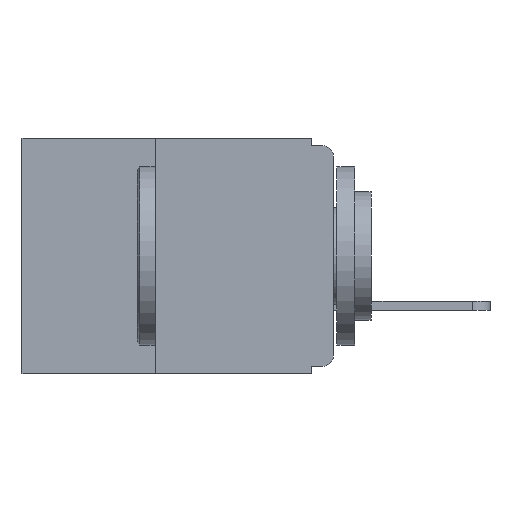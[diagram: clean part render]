
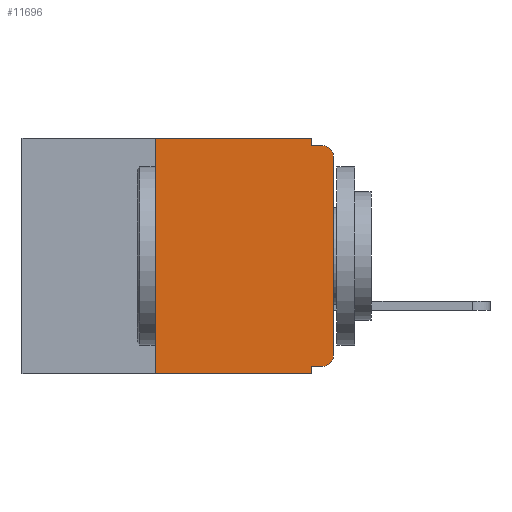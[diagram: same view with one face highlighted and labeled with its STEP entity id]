
A CAD part, left-side view. The second image highlights one B-rep face of the part: STEP entity #11696.
In plain terms, the highlighted planar face has unit normal (-1, 0, 0).
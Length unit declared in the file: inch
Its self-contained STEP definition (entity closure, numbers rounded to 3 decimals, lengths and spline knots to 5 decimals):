
#84 = EDGE_CURVE ( 'NONE', #11454, #4569, #12786, .T. ) ;
#391 = CARTESIAN_POINT ( 'NONE',  ( 0., 0., 0. ) ) ;
#518 = VECTOR ( 'NONE', #15742, 39.37008 ) ;
#551 = VERTEX_POINT ( 'NONE', #2414 ) ;
#1000 = LINE ( 'NONE', #11585, #13023 ) ;
#1158 = EDGE_CURVE ( 'NONE', #9826, #9682, #7906, .T. ) ;
#1329 = CARTESIAN_POINT ( 'NONE',  ( 0., 0.031, -0.33 ) ) ;
#1333 = VECTOR ( 'NONE', #4972, 39.37008 ) ;
#1735 = AXIS2_PLACEMENT_3D ( 'NONE', #10075, #7934, #3532 ) ;
#1920 = EDGE_CURVE ( 'NONE', #6484, #8667, #3217, .T. ) ;
#2244 = CARTESIAN_POINT ( 'NONE',  ( 0., 0., -0.32 ) ) ;
#2414 = CARTESIAN_POINT ( 'NONE',  ( 0., 0.25, -0.33 ) ) ;
#2590 = VECTOR ( 'NONE', #13302, 39.37008 ) ;
#3217 = CIRCLE ( 'NONE', #10642, 0.015 ) ;
#3390 = CARTESIAN_POINT ( 'NONE',  ( 0., 0.015, -0.32 ) ) ;
#3454 = EDGE_CURVE ( 'NONE', #6484, #11454, #14997, .T. ) ;
#3532 = DIRECTION ( 'NONE',  ( 0., 0., -1. ) ) ;
#4244 = DIRECTION ( 'NONE',  ( 0., 0., -1. ) ) ;
#4375 = ORIENTED_EDGE ( 'NONE', *, *, #4645, .F. ) ;
#4415 = CARTESIAN_POINT ( 'NONE',  ( 0., 0.015, -0.305 ) ) ;
#4519 = CARTESIAN_POINT ( 'NONE',  ( 0., 0.25, 0. ) ) ;
#4569 = VERTEX_POINT ( 'NONE', #1329 ) ;
#4645 = EDGE_CURVE ( 'NONE', #9682, #10896, #1000, .T. ) ;
#4791 = ORIENTED_EDGE ( 'NONE', *, *, #10527, .T. ) ;
#4972 = DIRECTION ( 'NONE',  ( 0., -1., 0. ) ) ;
#5139 = ORIENTED_EDGE ( 'NONE', *, *, #84, .F. ) ;
#6115 = LINE ( 'NONE', #10929, #11554 ) ;
#6153 = FACE_OUTER_BOUND ( 'NONE', #7063, .T. ) ;
#6484 = VERTEX_POINT ( 'NONE', #3390 ) ;
#6766 = CARTESIAN_POINT ( 'NONE',  ( 0., 0.437, -0.33 ) ) ;
#7063 = EDGE_LOOP ( 'NONE', ( #11499, #4791, #9771, #4375, #14673, #13803, #12579, #5139, #9735, #7335 ) ) ;
#7159 = DIRECTION ( 'NONE',  ( 0., 0., -1. ) ) ;
#7201 = PLANE ( 'NONE',  #1735 ) ;
#7335 = ORIENTED_EDGE ( 'NONE', *, *, #1920, .T. ) ;
#7432 = CARTESIAN_POINT ( 'NONE',  ( 0., 0.031, -0.33 ) ) ;
#7902 = DIRECTION ( 'NONE',  ( 0., -1., 0. ) ) ;
#7906 = LINE ( 'NONE', #10744, #518 ) ;
#7934 = DIRECTION ( 'NONE',  ( 1., 0., 0. ) ) ;
#7978 = VECTOR ( 'NONE', #13998, 39.37008 ) ;
#8246 = CARTESIAN_POINT ( 'NONE',  ( 0., 0.031, -0.01 ) ) ;
#8367 = DIRECTION ( 'NONE',  ( -1., 0., 0. ) ) ;
#8544 = CIRCLE ( 'NONE', #11048, 0.015 ) ;
#8584 = DIRECTION ( 'NONE',  ( 0., 0., 1. ) ) ;
#8633 = DIRECTION ( 'NONE',  ( 0., 0., -1. ) ) ;
#8667 = VERTEX_POINT ( 'NONE', #10790 ) ;
#8693 = CARTESIAN_POINT ( 'NONE',  ( 0., 0.015, -0.025 ) ) ;
#8848 = CARTESIAN_POINT ( 'NONE',  ( 0., 0., -0.01 ) ) ;
#9064 = CARTESIAN_POINT ( 'NONE',  ( 0., 0., -0.025 ) ) ;
#9523 = VECTOR ( 'NONE', #8633, 39.37008 ) ;
#9682 = VERTEX_POINT ( 'NONE', #15117 ) ;
#9735 = ORIENTED_EDGE ( 'NONE', *, *, #3454, .F. ) ;
#9771 = ORIENTED_EDGE ( 'NONE', *, *, #10522, .F. ) ;
#9826 = VERTEX_POINT ( 'NONE', #4519 ) ;
#9944 = DIRECTION ( 'NONE',  ( -1., 0., 0. ) ) ;
#10005 = EDGE_CURVE ( 'NONE', #8667, #11952, #14163, .T. ) ;
#10075 = CARTESIAN_POINT ( 'NONE',  ( 0., 0.437, 0. ) ) ;
#10522 = EDGE_CURVE ( 'NONE', #10896, #11429, #14916, .T. ) ;
#10527 = EDGE_CURVE ( 'NONE', #11952, #11429, #8544, .T. ) ;
#10573 = LINE ( 'NONE', #6766, #13062 ) ;
#10642 = AXIS2_PLACEMENT_3D ( 'NONE', #4415, #8367, #7159 ) ;
#10744 = CARTESIAN_POINT ( 'NONE',  ( 0., 0.437, 0. ) ) ;
#10790 = CARTESIAN_POINT ( 'NONE',  ( 0., 0., -0.305 ) ) ;
#10896 = VERTEX_POINT ( 'NONE', #8246 ) ;
#10929 = CARTESIAN_POINT ( 'NONE',  ( 0., 0.25, -0.33 ) ) ;
#11048 = AXIS2_PLACEMENT_3D ( 'NONE', #8693, #9944, #11182 ) ;
#11182 = DIRECTION ( 'NONE',  ( 0., 0., -1. ) ) ;
#11429 = VERTEX_POINT ( 'NONE', #12475 ) ;
#11454 = VERTEX_POINT ( 'NONE', #12737 ) ;
#11499 = ORIENTED_EDGE ( 'NONE', *, *, #10005, .T. ) ;
#11554 = VECTOR ( 'NONE', #8584, 39.37008 ) ;
#11585 = CARTESIAN_POINT ( 'NONE',  ( 0., 0.031, 0. ) ) ;
#11696 = ADVANCED_FACE ( 'NONE', ( #6153 ), #7201, .F. ) ;
#11952 = VERTEX_POINT ( 'NONE', #9064 ) ;
#12475 = CARTESIAN_POINT ( 'NONE',  ( 0., 0.015, -0.01 ) ) ;
#12579 = ORIENTED_EDGE ( 'NONE', *, *, #13864, .T. ) ;
#12737 = CARTESIAN_POINT ( 'NONE',  ( 0., 0.031, -0.32 ) ) ;
#12786 = LINE ( 'NONE', #7432, #9523 ) ;
#13023 = VECTOR ( 'NONE', #4244, 39.37008 ) ;
#13062 = VECTOR ( 'NONE', #7902, 39.37008 ) ;
#13164 = EDGE_CURVE ( 'NONE', #551, #9826, #6115, .T. ) ;
#13302 = DIRECTION ( 'NONE',  ( 0., 1., 0. ) ) ;
#13803 = ORIENTED_EDGE ( 'NONE', *, *, #13164, .F. ) ;
#13864 = EDGE_CURVE ( 'NONE', #551, #4569, #10573, .T. ) ;
#13998 = DIRECTION ( 'NONE',  ( 0., 0., 1. ) ) ;
#14163 = LINE ( 'NONE', #391, #7978 ) ;
#14673 = ORIENTED_EDGE ( 'NONE', *, *, #1158, .F. ) ;
#14916 = LINE ( 'NONE', #8848, #1333 ) ;
#14997 = LINE ( 'NONE', #2244, #2590 ) ;
#15117 = CARTESIAN_POINT ( 'NONE',  ( 0., 0.031, 0. ) ) ;
#15742 = DIRECTION ( 'NONE',  ( 0., -1., 0. ) ) ;
